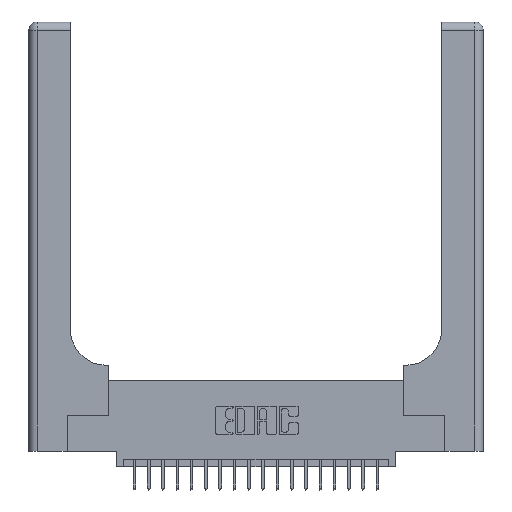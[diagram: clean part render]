
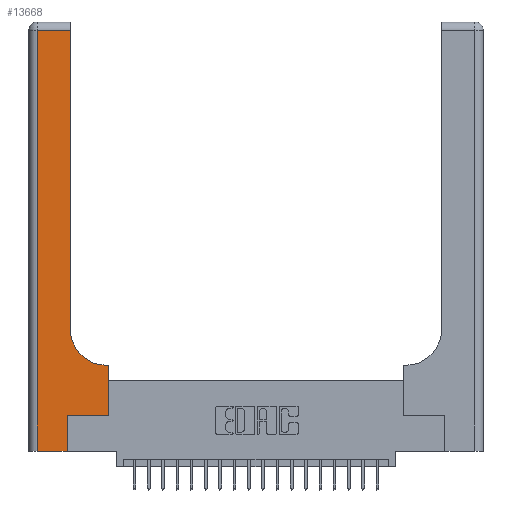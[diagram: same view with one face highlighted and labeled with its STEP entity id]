
A CAD part, top view. The second image highlights one B-rep face of the part: STEP entity #13668.
In plain terms, the highlighted planar face has unit normal (0, 0, 1).
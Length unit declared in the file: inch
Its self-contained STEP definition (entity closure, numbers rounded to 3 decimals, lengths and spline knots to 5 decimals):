
#490 = VERTEX_POINT ( 'NONE', #17784 ) ;
#1010 = ORIENTED_EDGE ( 'NONE', *, *, #3757, .T. ) ;
#2114 = CARTESIAN_POINT ( 'NONE',  ( 0.5585, 0.6, 0.37 ) ) ;
#2461 = VECTOR ( 'NONE', #10675, 39.37008 ) ;
#2551 = DIRECTION ( 'NONE',  ( 1., 0., 0. ) ) ;
#3209 = DIRECTION ( 'NONE',  ( 1., 0., 0. ) ) ;
#3352 = VERTEX_POINT ( 'NONE', #5960 ) ;
#3469 = LINE ( 'NONE', #16628, #6482 ) ;
#3757 = EDGE_CURVE ( 'NONE', #20043, #12481, #11999, .T. ) ;
#3792 = EDGE_CURVE ( 'NONE', #3352, #490, #3469, .T. ) ;
#3806 = DIRECTION ( 'NONE',  ( 1., 0., 0. ) ) ;
#3815 = CARTESIAN_POINT ( 'NONE',  ( 0.5585, 0.25, 0.37 ) ) ;
#4152 = ORIENTED_EDGE ( 'NONE', *, *, #6950, .T. ) ;
#4226 = ORIENTED_EDGE ( 'NONE', *, *, #15476, .T. ) ;
#4844 = CARTESIAN_POINT ( 'NONE',  ( 0.5585, 0.25, 0.37 ) ) ;
#4982 = EDGE_LOOP ( 'NONE', ( #1010, #4152, #4226, #15889, #6975, #8575, #19024, #5286, #20632 ) ) ;
#5286 = ORIENTED_EDGE ( 'NONE', *, *, #13139, .T. ) ;
#5329 = CARTESIAN_POINT ( 'NONE',  ( 0.2915, 3., 0.37 ) ) ;
#5478 = DIRECTION ( 'NONE',  ( 0., 1., 0. ) ) ;
#5718 = DIRECTION ( 'NONE',  ( -1., 0., 0. ) ) ;
#5960 = CARTESIAN_POINT ( 'NONE',  ( 0.06, 0., 0.37 ) ) ;
#6170 = CARTESIAN_POINT ( 'NONE',  ( 0.2915, 2.94, 0.37 ) ) ;
#6482 = VECTOR ( 'NONE', #2551, 39.37008 ) ;
#6950 = EDGE_CURVE ( 'NONE', #12481, #19307, #10735, .T. ) ;
#6975 = ORIENTED_EDGE ( 'NONE', *, *, #20248, .T. ) ;
#7139 = LINE ( 'NONE', #21044, #12389 ) ;
#7647 = CIRCLE ( 'NONE', #19292, 0.25 ) ;
#7847 = VECTOR ( 'NONE', #13464, 39.37008 ) ;
#7978 = CARTESIAN_POINT ( 'NONE',  ( 0.2915, 0.85, 0.37 ) ) ;
#8276 = EDGE_CURVE ( 'NONE', #21387, #11757, #16213, .T. ) ;
#8565 = DIRECTION ( 'NONE',  ( 0., 0., -1. ) ) ;
#8575 = ORIENTED_EDGE ( 'NONE', *, *, #11768, .T. ) ;
#8811 = DIRECTION ( 'NONE',  ( -1., 0., 0. ) ) ;
#9847 = DIRECTION ( 'NONE',  ( -1., 0., 0. ) ) ;
#9901 = VERTEX_POINT ( 'NONE', #11347 ) ;
#10003 = PLANE ( 'NONE',  #18848 ) ;
#10078 = DIRECTION ( 'NONE',  ( 0., 0., -1. ) ) ;
#10347 = VECTOR ( 'NONE', #5478, 39.37008 ) ;
#10479 = VECTOR ( 'NONE', #5718, 39.37008 ) ;
#10675 = DIRECTION ( 'NONE',  ( 0., 1., 0. ) ) ;
#10735 = LINE ( 'NONE', #18095, #10479 ) ;
#11347 = CARTESIAN_POINT ( 'NONE',  ( 0.269, 0.25, 0.37 ) ) ;
#11743 = VECTOR ( 'NONE', #13693, 39.37008 ) ;
#11757 = VERTEX_POINT ( 'NONE', #2114 ) ;
#11768 = EDGE_CURVE ( 'NONE', #9901, #21387, #19364, .T. ) ;
#11999 = LINE ( 'NONE', #5329, #10347 ) ;
#12389 = VECTOR ( 'NONE', #8811, 39.37008 ) ;
#12481 = VERTEX_POINT ( 'NONE', #6170 ) ;
#13139 = EDGE_CURVE ( 'NONE', #11757, #15373, #7139, .T. ) ;
#13464 = DIRECTION ( 'NONE',  ( 0., 1., 0. ) ) ;
#13668 = ADVANCED_FACE ( 'NONE', ( #21161 ), #10003, .F. ) ;
#13693 = DIRECTION ( 'NONE',  ( 0., -1., 0. ) ) ;
#14141 = CARTESIAN_POINT ( 'NONE',  ( 0.269, 0.25, 0.37 ) ) ;
#14235 = EDGE_CURVE ( 'NONE', #15373, #20043, #7647, .T. ) ;
#14662 = VECTOR ( 'NONE', #3806, 39.37008 ) ;
#15373 = VERTEX_POINT ( 'NONE', #22277 ) ;
#15476 = EDGE_CURVE ( 'NONE', #19307, #3352, #20802, .T. ) ;
#15520 = CARTESIAN_POINT ( 'NONE',  ( 0.5415, 0.85, 0.37 ) ) ;
#15889 = ORIENTED_EDGE ( 'NONE', *, *, #3792, .T. ) ;
#16213 = LINE ( 'NONE', #3815, #2461 ) ;
#16628 = CARTESIAN_POINT ( 'NONE',  ( 0., 0., 0.37 ) ) ;
#17075 = CARTESIAN_POINT ( 'NONE',  ( 0.269, 0., 0.37 ) ) ;
#17390 = CARTESIAN_POINT ( 'NONE',  ( 0.06, 3., 0.37 ) ) ;
#17784 = CARTESIAN_POINT ( 'NONE',  ( 0.269, 0., 0.37 ) ) ;
#18095 = CARTESIAN_POINT ( 'NONE',  ( 0., 2.94, 0.37 ) ) ;
#18848 = AXIS2_PLACEMENT_3D ( 'NONE', #20389, #10078, #9847 ) ;
#19024 = ORIENTED_EDGE ( 'NONE', *, *, #8276, .T. ) ;
#19292 = AXIS2_PLACEMENT_3D ( 'NONE', #15520, #8565, #3209 ) ;
#19307 = VERTEX_POINT ( 'NONE', #21829 ) ;
#19364 = LINE ( 'NONE', #14141, #14662 ) ;
#20043 = VERTEX_POINT ( 'NONE', #7978 ) ;
#20245 = LINE ( 'NONE', #17075, #7847 ) ;
#20248 = EDGE_CURVE ( 'NONE', #490, #9901, #20245, .T. ) ;
#20389 = CARTESIAN_POINT ( 'NONE',  ( 0., 3., 0.37 ) ) ;
#20632 = ORIENTED_EDGE ( 'NONE', *, *, #14235, .T. ) ;
#20802 = LINE ( 'NONE', #17390, #11743 ) ;
#21044 = CARTESIAN_POINT ( 'NONE',  ( 0.2915, 0.6, 0.37 ) ) ;
#21161 = FACE_OUTER_BOUND ( 'NONE', #4982, .T. ) ;
#21387 = VERTEX_POINT ( 'NONE', #4844 ) ;
#21829 = CARTESIAN_POINT ( 'NONE',  ( 0.06, 2.94, 0.37 ) ) ;
#22277 = CARTESIAN_POINT ( 'NONE',  ( 0.5415, 0.6, 0.37 ) ) ;
